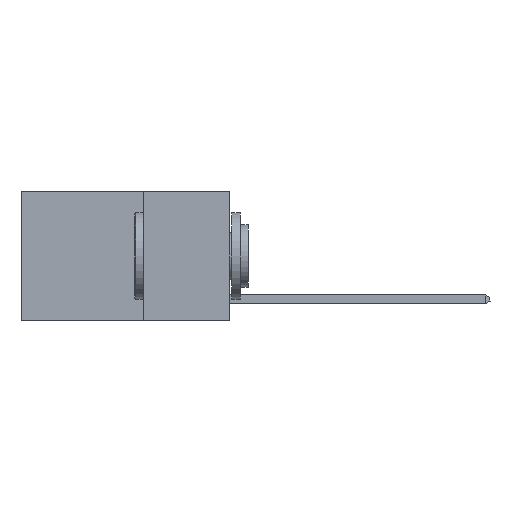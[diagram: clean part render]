
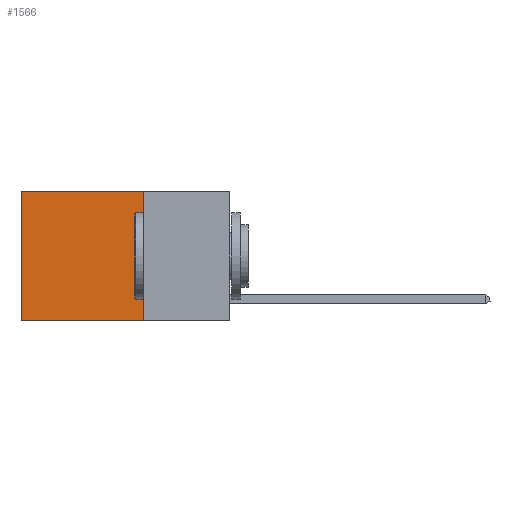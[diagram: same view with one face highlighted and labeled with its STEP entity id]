
A CAD part, left-side view. The second image highlights one B-rep face of the part: STEP entity #1566.
In plain terms, the highlighted planar face has unit normal (-1, 0, 0).
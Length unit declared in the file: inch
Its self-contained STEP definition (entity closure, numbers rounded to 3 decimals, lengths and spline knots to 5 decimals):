
#609 = EDGE_CURVE ( 'NONE', #3182, #2665, #3445, .T. ) ;
#1566 = ADVANCED_FACE ( 'NONE', ( #3869 ), #4982, .F. ) ;
#2362 = ORIENTED_EDGE ( 'NONE', *, *, #8527, .T. ) ;
#2426 = LINE ( 'NONE', #4697, #15445 ) ;
#2528 = VECTOR ( 'NONE', #12537, 39.37008 ) ;
#2563 = EDGE_CURVE ( 'NONE', #15465, #3182, #11565, .T. ) ;
#2665 = VERTEX_POINT ( 'NONE', #4537 ) ;
#2716 = VERTEX_POINT ( 'NONE', #6796 ) ;
#2805 = EDGE_CURVE ( 'NONE', #2716, #2665, #2426, .T. ) ;
#3182 = VERTEX_POINT ( 'NONE', #9713 ) ;
#3445 = LINE ( 'NONE', #7147, #10238 ) ;
#3869 = FACE_OUTER_BOUND ( 'NONE', #5322, .T. ) ;
#4537 = CARTESIAN_POINT ( 'NONE',  ( 0.2625, 0.6, -0.37 ) ) ;
#4697 = CARTESIAN_POINT ( 'NONE',  ( 0.2625, 0.6, 0. ) ) ;
#4982 = PLANE ( 'NONE',  #11561 ) ;
#5322 = EDGE_LOOP ( 'NONE', ( #10797, #8869, #13421, #2362 ) ) ;
#6602 = LINE ( 'NONE', #12740, #12261 ) ;
#6796 = CARTESIAN_POINT ( 'NONE',  ( 0.2625, 0.6, 0. ) ) ;
#6825 = DIRECTION ( 'NONE',  ( 0., 1., 0. ) ) ;
#7147 = CARTESIAN_POINT ( 'NONE',  ( 0.2625, 0.25, -0.37 ) ) ;
#8527 = EDGE_CURVE ( 'NONE', #15465, #2716, #6602, .T. ) ;
#8677 = CARTESIAN_POINT ( 'NONE',  ( 0.2625, 0.25, 0. ) ) ;
#8869 = ORIENTED_EDGE ( 'NONE', *, *, #609, .F. ) ;
#9713 = CARTESIAN_POINT ( 'NONE',  ( 0.2625, 0.25, -0.37 ) ) ;
#9974 = DIRECTION ( 'NONE',  ( 1., 0., 0. ) ) ;
#10238 = VECTOR ( 'NONE', #6825, 39.37008 ) ;
#10797 = ORIENTED_EDGE ( 'NONE', *, *, #2805, .T. ) ;
#11561 = AXIS2_PLACEMENT_3D ( 'NONE', #8677, #9974, #13618 ) ;
#11565 = LINE ( 'NONE', #12852, #2528 ) ;
#11752 = CARTESIAN_POINT ( 'NONE',  ( 0.2625, 0.25, 0. ) ) ;
#12261 = VECTOR ( 'NONE', #15014, 39.37008 ) ;
#12537 = DIRECTION ( 'NONE',  ( 0., 0., -1. ) ) ;
#12740 = CARTESIAN_POINT ( 'NONE',  ( 0.2625, 0.25, 0. ) ) ;
#12852 = CARTESIAN_POINT ( 'NONE',  ( 0.2625, 0.25, 0. ) ) ;
#13421 = ORIENTED_EDGE ( 'NONE', *, *, #2563, .F. ) ;
#13618 = DIRECTION ( 'NONE',  ( 0., 0., -1. ) ) ;
#14632 = DIRECTION ( 'NONE',  ( 0., 0., -1. ) ) ;
#15014 = DIRECTION ( 'NONE',  ( 0., 1., 0. ) ) ;
#15445 = VECTOR ( 'NONE', #14632, 39.37008 ) ;
#15465 = VERTEX_POINT ( 'NONE', #11752 ) ;
